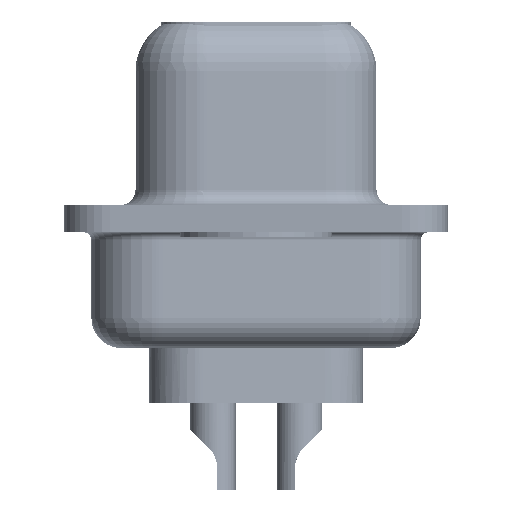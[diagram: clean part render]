
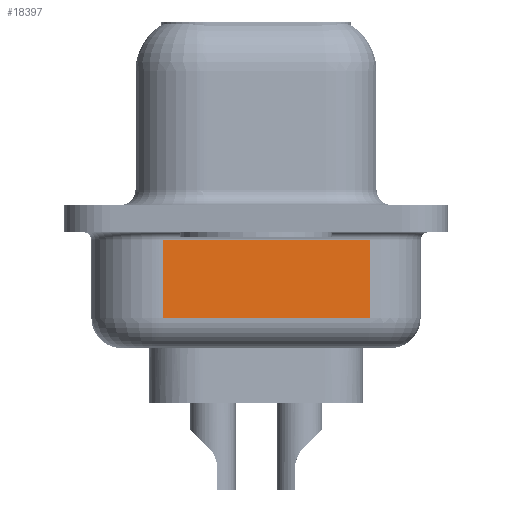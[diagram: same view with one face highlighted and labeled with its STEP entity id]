
A CAD part, left-side view. The second image highlights one B-rep face of the part: STEP entity #18397.
In plain terms, the highlighted planar face has unit normal (-0.985, -0.174, 0).
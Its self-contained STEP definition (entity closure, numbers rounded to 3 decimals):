
#899 = LINE ( 'NONE', #26646, #18547 ) ;
#1741 = ORIENTED_EDGE ( 'NONE', *, *, #5730, .T. ) ;
#2351 = EDGE_CURVE ( 'NONE', #10351, #6675, #899, .T. ) ;
#2916 = DIRECTION ( 'NONE',  ( -0.174, 0.985, 0. ) ) ;
#3577 = AXIS2_PLACEMENT_3D ( 'NONE', #11942, #20709, #20269 ) ;
#4145 = CARTESIAN_POINT ( 'NONE',  ( 4.079, -3.747, -0.7 ) ) ;
#5730 = EDGE_CURVE ( 'NONE', #17268, #13629, #27572, .T. ) ;
#5774 = DIRECTION ( 'NONE',  ( 0., 0., 1. ) ) ;
#6675 = VERTEX_POINT ( 'NONE', #15939 ) ;
#6983 = EDGE_LOOP ( 'NONE', ( #22707, #19774, #1741, #22048 ) ) ;
#9283 = VECTOR ( 'NONE', #11535, 1000. ) ;
#9796 = LINE ( 'NONE', #15989, #10805 ) ;
#10351 = VERTEX_POINT ( 'NONE', #26542 ) ;
#10805 = VECTOR ( 'NONE', #2916, 1000. ) ;
#11535 = DIRECTION ( 'NONE',  ( 0.174, -0.985, 0. ) ) ;
#11942 = CARTESIAN_POINT ( 'NONE',  ( 2.88, 3.053, -4.25 ) ) ;
#13629 = VERTEX_POINT ( 'NONE', #4145 ) ;
#13649 = CARTESIAN_POINT ( 'NONE',  ( 4.079, -3.747, -3.25 ) ) ;
#13657 = PLANE ( 'NONE',  #3577 ) ;
#13836 = CARTESIAN_POINT ( 'NONE',  ( 2.88, 3.053, -3.25 ) ) ;
#15797 = FACE_OUTER_BOUND ( 'NONE', #6983, .T. ) ;
#15939 = CARTESIAN_POINT ( 'NONE',  ( 2.88, 3.053, -0.7 ) ) ;
#15989 = CARTESIAN_POINT ( 'NONE',  ( 2.88, 3.053, -0.7 ) ) ;
#16631 = CARTESIAN_POINT ( 'NONE',  ( 4.079, -3.747, -4.25 ) ) ;
#17268 = VERTEX_POINT ( 'NONE', #13649 ) ;
#18397 = ADVANCED_FACE ( 'NONE', ( #15797 ), #13657, .F. ) ;
#18547 = VECTOR ( 'NONE', #5774, 1000. ) ;
#19774 = ORIENTED_EDGE ( 'NONE', *, *, #21395, .T. ) ;
#20269 = DIRECTION ( 'NONE',  ( -0.174, 0.985, 0. ) ) ;
#20709 = DIRECTION ( 'NONE',  ( 0.985, 0.174, 0. ) ) ;
#21395 = EDGE_CURVE ( 'NONE', #10351, #17268, #22477, .T. ) ;
#22048 = ORIENTED_EDGE ( 'NONE', *, *, #25041, .T. ) ;
#22477 = LINE ( 'NONE', #13836, #9283 ) ;
#22707 = ORIENTED_EDGE ( 'NONE', *, *, #2351, .F. ) ;
#25041 = EDGE_CURVE ( 'NONE', #13629, #6675, #9796, .T. ) ;
#25406 = DIRECTION ( 'NONE',  ( 0., 0., 1. ) ) ;
#25712 = VECTOR ( 'NONE', #25406, 1000. ) ;
#26542 = CARTESIAN_POINT ( 'NONE',  ( 2.88, 3.053, -3.25 ) ) ;
#26646 = CARTESIAN_POINT ( 'NONE',  ( 2.88, 3.053, -4.25 ) ) ;
#27572 = LINE ( 'NONE', #16631, #25712 ) ;
